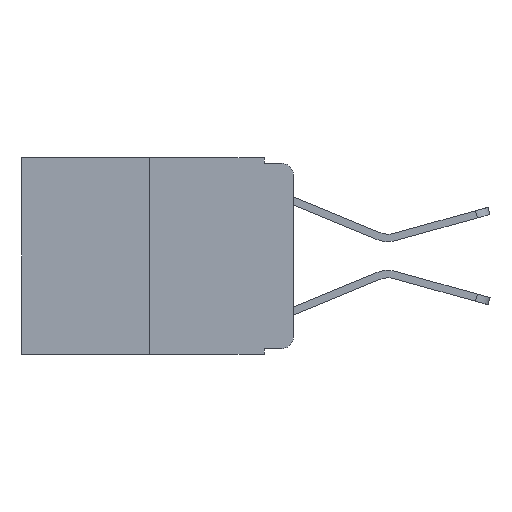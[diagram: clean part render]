
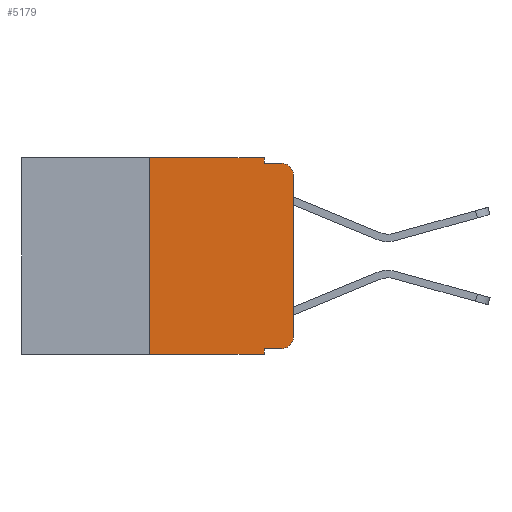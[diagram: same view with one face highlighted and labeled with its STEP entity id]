
A CAD part, left-side view. The second image highlights one B-rep face of the part: STEP entity #5179.
In plain terms, the highlighted planar face has unit normal (-1, 0, 0).
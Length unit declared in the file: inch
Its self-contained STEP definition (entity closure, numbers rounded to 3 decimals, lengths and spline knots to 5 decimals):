
#502 = AXIS2_PLACEMENT_3D ( 'NONE', #7540, #22438, #20572 ) ;
#512 = ORIENTED_EDGE ( 'NONE', *, *, #8125, .F. ) ;
#1036 = LINE ( 'NONE', #23632, #9774 ) ;
#1595 = CARTESIAN_POINT ( 'NONE',  ( 0., 0.051, -0.333 ) ) ;
#1802 = CIRCLE ( 'NONE', #502, 0.02 ) ;
#2020 = EDGE_CURVE ( 'NONE', #2184, #19145, #13730, .T. ) ;
#2176 = DIRECTION ( 'NONE',  ( 0., 0., -1. ) ) ;
#2184 = VERTEX_POINT ( 'NONE', #2258 ) ;
#2226 = EDGE_CURVE ( 'NONE', #4918, #6954, #4429, .T. ) ;
#2258 = CARTESIAN_POINT ( 'NONE',  ( 0., 0.051, -0.01 ) ) ;
#2818 = VERTEX_POINT ( 'NONE', #9599 ) ;
#3025 = AXIS2_PLACEMENT_3D ( 'NONE', #7626, #9512, #22908 ) ;
#3393 = DIRECTION ( 'NONE',  ( 0., 0., 1. ) ) ;
#3718 = ORIENTED_EDGE ( 'NONE', *, *, #12121, .T. ) ;
#3906 = VERTEX_POINT ( 'NONE', #20748 ) ;
#4200 = EDGE_CURVE ( 'NONE', #11420, #2184, #6063, .T. ) ;
#4209 = ORIENTED_EDGE ( 'NONE', *, *, #2020, .F. ) ;
#4429 = CIRCLE ( 'NONE', #3025, 0.02 ) ;
#4496 = VECTOR ( 'NONE', #4884, 39.37008 ) ;
#4884 = DIRECTION ( 'NONE',  ( 0., -1., 0. ) ) ;
#4918 = VERTEX_POINT ( 'NONE', #21673 ) ;
#4975 = LINE ( 'NONE', #5112, #5837 ) ;
#5009 = ORIENTED_EDGE ( 'NONE', *, *, #23778, .F. ) ;
#5040 = CARTESIAN_POINT ( 'NONE',  ( 0., 0., -0.03 ) ) ;
#5112 = CARTESIAN_POINT ( 'NONE',  ( 0., 0.051, 0. ) ) ;
#5179 = ADVANCED_FACE ( 'NONE', ( #6928 ), #22468, .F. ) ;
#5192 = DIRECTION ( 'NONE',  ( 0., 0., -1. ) ) ;
#5762 = DIRECTION ( 'NONE',  ( 0., -1., 0. ) ) ;
#5837 = VECTOR ( 'NONE', #6992, 39.37008 ) ;
#5920 = VECTOR ( 'NONE', #3393, 39.37008 ) ;
#6063 = LINE ( 'NONE', #16256, #23842 ) ;
#6928 = FACE_OUTER_BOUND ( 'NONE', #10699, .T. ) ;
#6954 = VERTEX_POINT ( 'NONE', #18040 ) ;
#6992 = DIRECTION ( 'NONE',  ( 0., 0., -1. ) ) ;
#7140 = CARTESIAN_POINT ( 'NONE',  ( 0., 0.25, 0. ) ) ;
#7540 = CARTESIAN_POINT ( 'NONE',  ( 0., 0.02, -0.03 ) ) ;
#7626 = CARTESIAN_POINT ( 'NONE',  ( 0., 0.02, -0.313 ) ) ;
#8125 = EDGE_CURVE ( 'NONE', #22913, #3906, #21372, .T. ) ;
#8340 = CARTESIAN_POINT ( 'NONE',  ( 0., 0., 0. ) ) ;
#8567 = CARTESIAN_POINT ( 'NONE',  ( 0., 0.051, -0.333 ) ) ;
#9512 = DIRECTION ( 'NONE',  ( -1., 0., 0. ) ) ;
#9599 = CARTESIAN_POINT ( 'NONE',  ( 0., 0.051, -0.343 ) ) ;
#9613 = DIRECTION ( 'NONE',  ( 1., 0., 0. ) ) ;
#9683 = CARTESIAN_POINT ( 'NONE',  ( 0., 0.473, 0. ) ) ;
#9774 = VECTOR ( 'NONE', #21854, 39.37008 ) ;
#9781 = LINE ( 'NONE', #8340, #16791 ) ;
#10699 = EDGE_LOOP ( 'NONE', ( #20770, #3718, #4209, #23354, #5009, #512, #19584, #18044, #18874, #18986 ) ) ;
#10809 = DIRECTION ( 'NONE',  ( 0., -1., 0. ) ) ;
#11420 = VERTEX_POINT ( 'NONE', #20199 ) ;
#12121 = EDGE_CURVE ( 'NONE', #20167, #19145, #1802, .T. ) ;
#12388 = LINE ( 'NONE', #8567, #4496 ) ;
#13730 = LINE ( 'NONE', #16909, #23961 ) ;
#13945 = DIRECTION ( 'NONE',  ( 0., 0., 1. ) ) ;
#15066 = LINE ( 'NONE', #17957, #20924 ) ;
#16256 = CARTESIAN_POINT ( 'NONE',  ( 0., 0.051, 0. ) ) ;
#16712 = EDGE_CURVE ( 'NONE', #22913, #2818, #1036, .T. ) ;
#16791 = VECTOR ( 'NONE', #13945, 39.37008 ) ;
#16909 = CARTESIAN_POINT ( 'NONE',  ( 0., 0.051, -0.01 ) ) ;
#16956 = CARTESIAN_POINT ( 'NONE',  ( 0., 0.02, -0.01 ) ) ;
#17957 = CARTESIAN_POINT ( 'NONE',  ( 0., 0.473, 0. ) ) ;
#18040 = CARTESIAN_POINT ( 'NONE',  ( 0., 0., -0.313 ) ) ;
#18044 = ORIENTED_EDGE ( 'NONE', *, *, #21866, .F. ) ;
#18071 = VERTEX_POINT ( 'NONE', #1595 ) ;
#18831 = EDGE_CURVE ( 'NONE', #6954, #20167, #9781, .T. ) ;
#18874 = ORIENTED_EDGE ( 'NONE', *, *, #19626, .T. ) ;
#18986 = ORIENTED_EDGE ( 'NONE', *, *, #2226, .T. ) ;
#19139 = AXIS2_PLACEMENT_3D ( 'NONE', #9683, #9613, #2176 ) ;
#19145 = VERTEX_POINT ( 'NONE', #16956 ) ;
#19584 = ORIENTED_EDGE ( 'NONE', *, *, #16712, .T. ) ;
#19626 = EDGE_CURVE ( 'NONE', #18071, #4918, #12388, .T. ) ;
#20167 = VERTEX_POINT ( 'NONE', #5040 ) ;
#20199 = CARTESIAN_POINT ( 'NONE',  ( 0., 0.051, 0. ) ) ;
#20572 = DIRECTION ( 'NONE',  ( 0., 0., -1. ) ) ;
#20748 = CARTESIAN_POINT ( 'NONE',  ( 0., 0.25, 0. ) ) ;
#20770 = ORIENTED_EDGE ( 'NONE', *, *, #18831, .T. ) ;
#20924 = VECTOR ( 'NONE', #10809, 39.37008 ) ;
#21162 = CARTESIAN_POINT ( 'NONE',  ( 0., 0.25, -0.343 ) ) ;
#21372 = LINE ( 'NONE', #7140, #5920 ) ;
#21673 = CARTESIAN_POINT ( 'NONE',  ( 0., 0.02, -0.333 ) ) ;
#21854 = DIRECTION ( 'NONE',  ( 0., -1., 0. ) ) ;
#21866 = EDGE_CURVE ( 'NONE', #18071, #2818, #4975, .T. ) ;
#22438 = DIRECTION ( 'NONE',  ( -1., 0., 0. ) ) ;
#22468 = PLANE ( 'NONE',  #19139 ) ;
#22908 = DIRECTION ( 'NONE',  ( 0., 0., -1. ) ) ;
#22913 = VERTEX_POINT ( 'NONE', #21162 ) ;
#23354 = ORIENTED_EDGE ( 'NONE', *, *, #4200, .F. ) ;
#23632 = CARTESIAN_POINT ( 'NONE',  ( 0., 0.473, -0.343 ) ) ;
#23778 = EDGE_CURVE ( 'NONE', #3906, #11420, #15066, .T. ) ;
#23842 = VECTOR ( 'NONE', #5192, 39.37008 ) ;
#23961 = VECTOR ( 'NONE', #5762, 39.37008 ) ;
